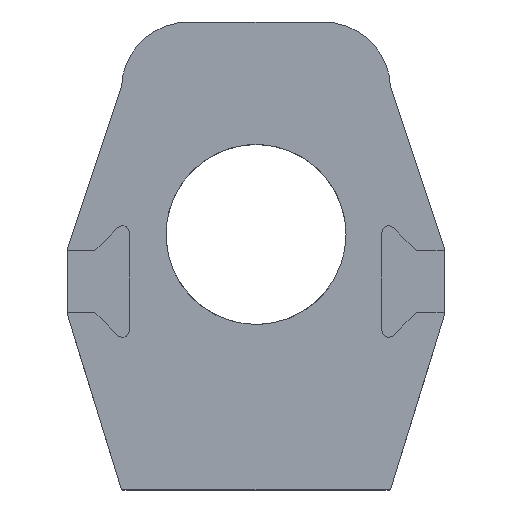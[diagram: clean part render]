
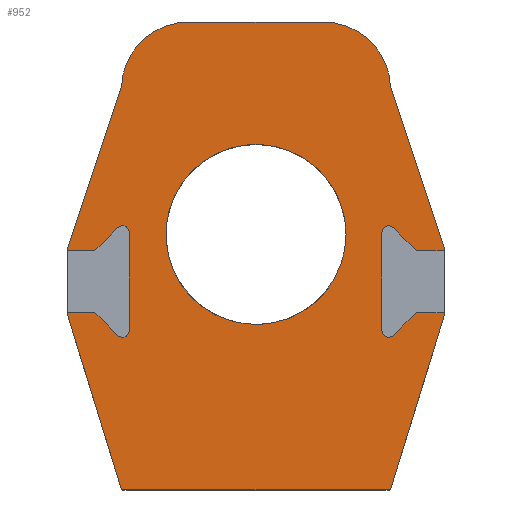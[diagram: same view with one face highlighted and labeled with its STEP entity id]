
A CAD part, front view. The second image highlights one B-rep face of the part: STEP entity #952.
In plain terms, the highlighted planar face has unit normal (0, -1, 0).
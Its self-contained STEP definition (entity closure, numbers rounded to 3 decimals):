
#19=ELLIPSE('',#1026,3.676,2.54);
#20=ELLIPSE('',#1027,3.676,2.54);
#58=FACE_BOUND('',#143,.T.);
#68=CIRCLE('',#1024,0.639);
#69=CIRCLE('',#1025,0.639);
#70=CIRCLE('',#1028,0.639);
#71=CIRCLE('',#1029,0.639);
#72=CIRCLE('',#1030,6.35);
#73=CIRCLE('',#1031,6.35);
#74=CIRCLE('',#1032,8.5);
#75=CIRCLE('',#1033,8.5);
#91=FACE_OUTER_BOUND('',#142,.T.);
#142=EDGE_LOOP('',(#661,#662,#663,#664,#665,#666,#667,#668,#669,#670,#671,
#672,#673,#674,#675,#676,#677,#678,#679,#680,#681,#682,#683,#684,#685,#686,
#687,#688));
#143=EDGE_LOOP('',(#689,#690));
#191=LINE('',#1397,#291);
#195=LINE('',#1405,#295);
#209=LINE('',#1448,#309);
#210=LINE('',#1450,#310);
#211=LINE('',#1454,#311);
#212=LINE('',#1458,#312);
#213=LINE('',#1459,#313);
#214=LINE('',#1461,#314);
#215=LINE('',#1465,#315);
#216=LINE('',#1469,#316);
#217=LINE('',#1471,#317);
#218=LINE('',#1473,#318);
#219=LINE('',#1475,#319);
#220=LINE('',#1479,#320);
#221=LINE('',#1483,#321);
#222=LINE('',#1485,#322);
#223=LINE('',#1487,#323);
#224=LINE('',#1489,#324);
#225=LINE('',#1493,#325);
#226=LINE('',#1496,#326);
#291=VECTOR('',#1109,10.);
#295=VECTOR('',#1113,10.);
#309=VECTOR('',#1149,10.);
#310=VECTOR('',#1150,10.);
#311=VECTOR('',#1153,10.);
#312=VECTOR('',#1156,10.);
#313=VECTOR('',#1157,10.);
#314=VECTOR('',#1158,10.);
#315=VECTOR('',#1161,10.);
#316=VECTOR('',#1164,10.);
#317=VECTOR('',#1165,10.);
#318=VECTOR('',#1166,10.);
#319=VECTOR('',#1167,10.);
#320=VECTOR('',#1170,10.);
#321=VECTOR('',#1173,10.);
#322=VECTOR('',#1174,10.);
#323=VECTOR('',#1175,10.);
#324=VECTOR('',#1176,10.);
#325=VECTOR('',#1179,10.);
#326=VECTOR('',#1182,10.);
#391=VERTEX_POINT('',#1395);
#392=VERTEX_POINT('',#1396);
#395=VERTEX_POINT('',#1402);
#396=VERTEX_POINT('',#1404);
#414=VERTEX_POINT('',#1447);
#415=VERTEX_POINT('',#1449);
#416=VERTEX_POINT('',#1451);
#417=VERTEX_POINT('',#1453);
#418=VERTEX_POINT('',#1455);
#419=VERTEX_POINT('',#1457);
#420=VERTEX_POINT('',#1460);
#421=VERTEX_POINT('',#1462);
#422=VERTEX_POINT('',#1464);
#423=VERTEX_POINT('',#1466);
#424=VERTEX_POINT('',#1468);
#425=VERTEX_POINT('',#1470);
#426=VERTEX_POINT('',#1472);
#427=VERTEX_POINT('',#1474);
#428=VERTEX_POINT('',#1476);
#429=VERTEX_POINT('',#1478);
#430=VERTEX_POINT('',#1480);
#431=VERTEX_POINT('',#1482);
#432=VERTEX_POINT('',#1484);
#433=VERTEX_POINT('',#1486);
#434=VERTEX_POINT('',#1488);
#435=VERTEX_POINT('',#1490);
#436=VERTEX_POINT('',#1492);
#437=VERTEX_POINT('',#1494);
#438=VERTEX_POINT('',#1497);
#439=VERTEX_POINT('',#1498);
#486=EDGE_CURVE('',#391,#392,#191,.T.);
#490=EDGE_CURVE('',#395,#396,#195,.T.);
#511=EDGE_CURVE('',#414,#392,#209,.T.);
#512=EDGE_CURVE('',#415,#414,#210,.T.);
#513=EDGE_CURVE('',#416,#415,#68,.T.);
#514=EDGE_CURVE('',#417,#416,#211,.T.);
#515=EDGE_CURVE('',#418,#417,#69,.T.);
#516=EDGE_CURVE('',#419,#418,#212,.T.);
#517=EDGE_CURVE('',#396,#419,#213,.T.);
#518=EDGE_CURVE('',#395,#420,#214,.T.);
#519=EDGE_CURVE('',#421,#420,#19,.T.);
#520=EDGE_CURVE('',#421,#422,#215,.T.);
#521=EDGE_CURVE('',#423,#422,#20,.T.);
#522=EDGE_CURVE('',#423,#424,#216,.T.);
#523=EDGE_CURVE('',#425,#424,#217,.T.);
#524=EDGE_CURVE('',#426,#425,#218,.T.);
#525=EDGE_CURVE('',#427,#426,#219,.T.);
#526=EDGE_CURVE('',#428,#427,#70,.T.);
#527=EDGE_CURVE('',#429,#428,#220,.T.);
#528=EDGE_CURVE('',#430,#429,#71,.T.);
#529=EDGE_CURVE('',#431,#430,#221,.T.);
#530=EDGE_CURVE('',#432,#431,#222,.T.);
#531=EDGE_CURVE('',#433,#432,#223,.T.);
#532=EDGE_CURVE('',#433,#434,#224,.T.);
#533=EDGE_CURVE('',#434,#435,#72,.T.);
#534=EDGE_CURVE('',#435,#436,#225,.T.);
#535=EDGE_CURVE('',#436,#437,#73,.T.);
#536=EDGE_CURVE('',#437,#391,#226,.T.);
#537=EDGE_CURVE('',#438,#439,#74,.T.);
#538=EDGE_CURVE('',#439,#438,#75,.T.);
#661=ORIENTED_EDGE('',*,*,#486,.T.);
#662=ORIENTED_EDGE('',*,*,#511,.F.);
#663=ORIENTED_EDGE('',*,*,#512,.F.);
#664=ORIENTED_EDGE('',*,*,#513,.F.);
#665=ORIENTED_EDGE('',*,*,#514,.F.);
#666=ORIENTED_EDGE('',*,*,#515,.F.);
#667=ORIENTED_EDGE('',*,*,#516,.F.);
#668=ORIENTED_EDGE('',*,*,#517,.F.);
#669=ORIENTED_EDGE('',*,*,#490,.F.);
#670=ORIENTED_EDGE('',*,*,#518,.T.);
#671=ORIENTED_EDGE('',*,*,#519,.F.);
#672=ORIENTED_EDGE('',*,*,#520,.T.);
#673=ORIENTED_EDGE('',*,*,#521,.F.);
#674=ORIENTED_EDGE('',*,*,#522,.T.);
#675=ORIENTED_EDGE('',*,*,#523,.F.);
#676=ORIENTED_EDGE('',*,*,#524,.F.);
#677=ORIENTED_EDGE('',*,*,#525,.F.);
#678=ORIENTED_EDGE('',*,*,#526,.F.);
#679=ORIENTED_EDGE('',*,*,#527,.F.);
#680=ORIENTED_EDGE('',*,*,#528,.F.);
#681=ORIENTED_EDGE('',*,*,#529,.F.);
#682=ORIENTED_EDGE('',*,*,#530,.F.);
#683=ORIENTED_EDGE('',*,*,#531,.F.);
#684=ORIENTED_EDGE('',*,*,#532,.T.);
#685=ORIENTED_EDGE('',*,*,#533,.T.);
#686=ORIENTED_EDGE('',*,*,#534,.T.);
#687=ORIENTED_EDGE('',*,*,#535,.T.);
#688=ORIENTED_EDGE('',*,*,#536,.T.);
#689=ORIENTED_EDGE('',*,*,#537,.T.);
#690=ORIENTED_EDGE('',*,*,#538,.T.);
#923=PLANE('',#1023);
#952=ADVANCED_FACE('',(#91,#58),#923,.F.);
#1023=AXIS2_PLACEMENT_3D('',#1446,#1147,#1148);
#1024=AXIS2_PLACEMENT_3D('',#1452,#1151,#1152);
#1025=AXIS2_PLACEMENT_3D('',#1456,#1154,#1155);
#1026=AXIS2_PLACEMENT_3D('',#1463,#1159,#1160);
#1027=AXIS2_PLACEMENT_3D('',#1467,#1162,#1163);
#1028=AXIS2_PLACEMENT_3D('',#1477,#1168,#1169);
#1029=AXIS2_PLACEMENT_3D('',#1481,#1171,#1172);
#1030=AXIS2_PLACEMENT_3D('',#1491,#1177,#1178);
#1031=AXIS2_PLACEMENT_3D('',#1495,#1180,#1181);
#1032=AXIS2_PLACEMENT_3D('',#1499,#1183,#1184);
#1033=AXIS2_PLACEMENT_3D('',#1500,#1185,#1186);
#1109=DIRECTION('',(0.,0.,-1.));
#1113=DIRECTION('',(0.,0.,1.));
#1147=DIRECTION('center_axis',(0.,1.,0.));
#1148=DIRECTION('ref_axis',(-1.,0.,0.));
#1149=DIRECTION('',(-1.,0.,-0.001));
#1150=DIRECTION('',(-0.707,0.,-0.707));
#1151=DIRECTION('center_axis',(0.,-1.,0.));
#1152=DIRECTION('ref_axis',(-0.707,0.,0.707));
#1153=DIRECTION('',(0.,0.,1.));
#1154=DIRECTION('center_axis',(0.,-1.,0.));
#1155=DIRECTION('ref_axis',(1.,0.,0.));
#1156=DIRECTION('',(0.707,0.,-0.707));
#1157=DIRECTION('',(1.,0.,0.));
#1158=DIRECTION('',(0.294,0.,-0.956));
#1159=DIRECTION('center_axis',(0.,1.,0.));
#1160=DIRECTION('ref_axis',(0.294,0.,-0.956));
#1161=DIRECTION('',(1.,0.,0.));
#1162=DIRECTION('center_axis',(0.,1.,0.));
#1163=DIRECTION('ref_axis',(-0.294,0.,-0.956));
#1164=DIRECTION('',(0.294,0.,0.956));
#1165=DIRECTION('',(0.,0.,-1.));
#1166=DIRECTION('',(1.,0.,0.));
#1167=DIRECTION('',(0.707,0.,0.707));
#1168=DIRECTION('center_axis',(0.,-1.,0.));
#1169=DIRECTION('ref_axis',(0.707,0.,-0.707));
#1170=DIRECTION('',(0.,0.,-1.));
#1171=DIRECTION('center_axis',(0.,-1.,0.));
#1172=DIRECTION('ref_axis',(-1.,0.,0.));
#1173=DIRECTION('',(-0.707,0.,0.707));
#1174=DIRECTION('',(-1.,0.,0.001));
#1175=DIRECTION('',(0.,0.,-1.));
#1176=DIRECTION('',(-0.316,0.,0.949));
#1177=DIRECTION('center_axis',(0.,-1.,0.));
#1178=DIRECTION('ref_axis',(0.999,0.,0.04));
#1179=DIRECTION('',(-1.,0.,0.));
#1180=DIRECTION('center_axis',(0.,-1.,0.));
#1181=DIRECTION('ref_axis',(-0.999,0.,0.04));
#1182=DIRECTION('',(-0.316,0.,-0.949));
#1183=DIRECTION('center_axis',(0.,1.,0.));
#1184=DIRECTION('ref_axis',(-1.,0.,0.));
#1185=DIRECTION('center_axis',(0.,1.,0.));
#1186=DIRECTION('ref_axis',(-1.,0.,0.));
#1395=CARTESIAN_POINT('',(-17.78,171.04,10.16));
#1396=CARTESIAN_POINT('',(-17.78,171.04,9.91));
#1397=CARTESIAN_POINT('',(-17.78,171.04,5.08));
#1402=CARTESIAN_POINT('',(-17.78,171.04,3.81));
#1404=CARTESIAN_POINT('',(-17.78,171.04,4.06));
#1405=CARTESIAN_POINT('',(-17.78,171.04,5.08));
#1446=CARTESIAN_POINT('Origin',(0.,171.04,6.35));
#1447=CARTESIAN_POINT('',(-15.214,171.04,9.913));
#1448=CARTESIAN_POINT('',(-8.892,171.04,9.921));
#1449=CARTESIAN_POINT('',(-13.066,171.04,12.061));
#1450=CARTESIAN_POINT('',(-12.265,171.04,12.862));
#1451=CARTESIAN_POINT('',(-11.975,171.04,11.609));
#1452=CARTESIAN_POINT('Origin',(-12.614,171.04,11.609));
#1453=CARTESIAN_POINT('',(-11.975,171.04,2.364));
#1454=CARTESIAN_POINT('',(-11.975,171.04,8.979));
#1455=CARTESIAN_POINT('',(-13.066,171.04,1.912));
#1456=CARTESIAN_POINT('Origin',(-12.614,171.04,2.364));
#1457=CARTESIAN_POINT('',(-15.214,171.04,4.06));
#1458=CARTESIAN_POINT('',(-10.909,171.04,-0.245));
#1459=CARTESIAN_POINT('',(-7.659,171.04,4.06));
#1460=CARTESIAN_POINT('',(-12.794,171.04,-12.394));
#1461=CARTESIAN_POINT('',(-14.828,171.04,-5.784));
#1462=CARTESIAN_POINT('',(-12.69,171.04,-12.699));
#1463=CARTESIAN_POINT('Origin',(-10.366,171.04,-11.647));
#1464=CARTESIAN_POINT('',(12.69,171.04,-12.699));
#1465=CARTESIAN_POINT('',(6.35,171.04,-12.699));
#1466=CARTESIAN_POINT('',(12.794,171.04,-12.394));
#1467=CARTESIAN_POINT('Origin',(10.366,171.04,-11.647));
#1468=CARTESIAN_POINT('',(17.78,171.04,3.81));
#1469=CARTESIAN_POINT('',(17.368,171.04,2.471));
#1470=CARTESIAN_POINT('',(17.78,171.04,4.06));
#1471=CARTESIAN_POINT('',(17.78,171.04,8.255));
#1472=CARTESIAN_POINT('',(15.136,171.04,4.06));
#1473=CARTESIAN_POINT('',(8.89,171.04,4.06));
#1474=CARTESIAN_POINT('',(12.989,171.04,1.912));
#1475=CARTESIAN_POINT('',(11.888,171.04,0.812));
#1476=CARTESIAN_POINT('',(11.898,171.04,2.364));
#1477=CARTESIAN_POINT('Origin',(12.537,171.04,2.364));
#1478=CARTESIAN_POINT('',(11.898,171.04,11.609));
#1479=CARTESIAN_POINT('',(11.898,171.04,4.357));
#1480=CARTESIAN_POINT('',(12.989,171.04,12.061));
#1481=CARTESIAN_POINT('Origin',(12.537,171.04,11.609));
#1482=CARTESIAN_POINT('',(15.136,171.04,9.913));
#1483=CARTESIAN_POINT('',(11.169,171.04,13.88));
#1484=CARTESIAN_POINT('',(17.78,171.04,9.91));
#1485=CARTESIAN_POINT('',(7.622,171.04,9.922));
#1486=CARTESIAN_POINT('',(17.78,171.04,10.16));
#1487=CARTESIAN_POINT('',(17.78,171.04,8.255));
#1488=CARTESIAN_POINT('',(12.7,171.04,25.4));
#1489=CARTESIAN_POINT('',(14.923,171.04,18.733));
#1490=CARTESIAN_POINT('',(6.355,171.04,31.496));
#1491=CARTESIAN_POINT('Origin',(6.355,171.04,25.146));
#1492=CARTESIAN_POINT('',(-6.355,171.04,31.496));
#1493=CARTESIAN_POINT('',(-6.35,171.04,31.496));
#1494=CARTESIAN_POINT('',(-12.7,171.04,25.4));
#1495=CARTESIAN_POINT('Origin',(-6.355,171.04,25.146));
#1496=CARTESIAN_POINT('',(-17.463,171.04,11.113));
#1497=CARTESIAN_POINT('',(8.064,171.04,14.118));
#1498=CARTESIAN_POINT('',(8.5,171.04,11.43));
#1499=CARTESIAN_POINT('Origin',(0.,171.04,11.43));
#1500=CARTESIAN_POINT('Origin',(0.,171.04,11.43));
